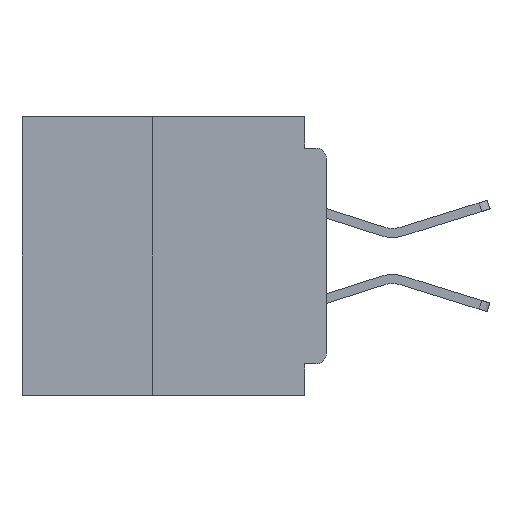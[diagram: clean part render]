
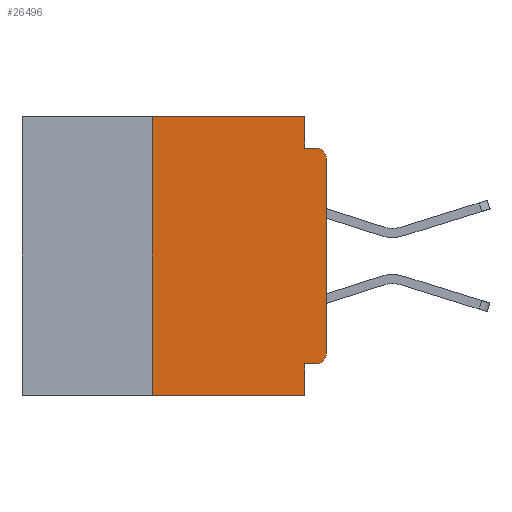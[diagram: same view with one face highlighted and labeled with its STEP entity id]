
A CAD part, left-side view. The second image highlights one B-rep face of the part: STEP entity #26496.
In plain terms, the highlighted planar face has unit normal (-1, 0, 0).
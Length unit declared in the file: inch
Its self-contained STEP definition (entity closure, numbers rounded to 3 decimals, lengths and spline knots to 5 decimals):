
#781 = LINE ( 'NONE', #15018, #24792 ) ;
#829 = CARTESIAN_POINT ( 'NONE',  ( 0., 0.015, -0.355 ) ) ;
#1220 = CARTESIAN_POINT ( 'NONE',  ( 0., 0.437, 0. ) ) ;
#1886 = EDGE_CURVE ( 'NONE', #57161, #25833, #57017, .T. ) ;
#2652 = CARTESIAN_POINT ( 'NONE',  ( 0., 0., -0.06 ) ) ;
#2807 = VERTEX_POINT ( 'NONE', #42373 ) ;
#3463 = ORIENTED_EDGE ( 'NONE', *, *, #7537, .F. ) ;
#3884 = CIRCLE ( 'NONE', #36840, 0.015 ) ;
#4123 = ORIENTED_EDGE ( 'NONE', *, *, #7112, .F. ) ;
#4292 = LINE ( 'NONE', #39189, #39430 ) ;
#5051 = CARTESIAN_POINT ( 'NONE',  ( 0., 0.031, -0.045 ) ) ;
#5560 = CARTESIAN_POINT ( 'NONE',  ( 0., 0.015, -0.34 ) ) ;
#5976 = VECTOR ( 'NONE', #29916, 39.37008 ) ;
#6452 = ORIENTED_EDGE ( 'NONE', *, *, #53035, .F. ) ;
#7112 = EDGE_CURVE ( 'NONE', #24129, #18933, #29905, .T. ) ;
#7407 = CARTESIAN_POINT ( 'NONE',  ( 0., 0., -0.34 ) ) ;
#7537 = EDGE_CURVE ( 'NONE', #20228, #24129, #18692, .T. ) ;
#7845 = PLANE ( 'NONE',  #27998 ) ;
#8189 = EDGE_CURVE ( 'NONE', #18933, #37794, #9601, .T. ) ;
#8416 = DIRECTION ( 'NONE',  ( 0., -1., 0. ) ) ;
#9601 = LINE ( 'NONE', #18985, #60178 ) ;
#9616 = LINE ( 'NONE', #17399, #20852 ) ;
#10145 = AXIS2_PLACEMENT_3D ( 'NONE', #24481, #25590, #25504 ) ;
#10401 = DIRECTION ( 'NONE',  ( 0., 0., -1. ) ) ;
#11096 = VECTOR ( 'NONE', #8416, 39.37008 ) ;
#11601 = EDGE_CURVE ( 'NONE', #55107, #50254, #9616, .T. ) ;
#13464 = CARTESIAN_POINT ( 'NONE',  ( 0., 0.437, -0.4 ) ) ;
#15018 = CARTESIAN_POINT ( 'NONE',  ( 0., 0., -0.045 ) ) ;
#15462 = DIRECTION ( 'NONE',  ( 0., 0., -1. ) ) ;
#15678 = ORIENTED_EDGE ( 'NONE', *, *, #1886, .T. ) ;
#16111 = ORIENTED_EDGE ( 'NONE', *, *, #24464, .F. ) ;
#17399 = CARTESIAN_POINT ( 'NONE',  ( 0., 0., -0.355 ) ) ;
#18692 = LINE ( 'NONE', #18847, #55066 ) ;
#18706 = ORIENTED_EDGE ( 'NONE', *, *, #11601, .F. ) ;
#18847 = CARTESIAN_POINT ( 'NONE',  ( 0., 0.25, -0.4 ) ) ;
#18933 = VERTEX_POINT ( 'NONE', #34058 ) ;
#18985 = CARTESIAN_POINT ( 'NONE',  ( 0., 0.031, 0. ) ) ;
#20228 = VERTEX_POINT ( 'NONE', #53778 ) ;
#20852 = VECTOR ( 'NONE', #41075, 39.37008 ) ;
#21966 = CARTESIAN_POINT ( 'NONE',  ( 0., 0.015, -0.045 ) ) ;
#22291 = LINE ( 'NONE', #13464, #11096 ) ;
#22297 = DIRECTION ( 'NONE',  ( 0., 0., -1. ) ) ;
#23599 = VECTOR ( 'NONE', #60745, 39.37008 ) ;
#24129 = VERTEX_POINT ( 'NONE', #32144 ) ;
#24464 = EDGE_CURVE ( 'NONE', #50254, #2807, #4292, .T. ) ;
#24481 = CARTESIAN_POINT ( 'NONE',  ( 0., 0.015, -0.06 ) ) ;
#24792 = VECTOR ( 'NONE', #53025, 39.37008 ) ;
#25103 = LINE ( 'NONE', #37173, #23599 ) ;
#25504 = DIRECTION ( 'NONE',  ( 0., 0., -1. ) ) ;
#25590 = DIRECTION ( 'NONE',  ( -1., 0., 0. ) ) ;
#25833 = VERTEX_POINT ( 'NONE', #21966 ) ;
#26496 = ADVANCED_FACE ( 'NONE', ( #38410 ), #7845, .F. ) ;
#27998 = AXIS2_PLACEMENT_3D ( 'NONE', #45972, #50729, #22297 ) ;
#28342 = EDGE_CURVE ( 'NONE', #55107, #53320, #3884, .T. ) ;
#28406 = ORIENTED_EDGE ( 'NONE', *, *, #28342, .T. ) ;
#29905 = LINE ( 'NONE', #1220, #5976 ) ;
#29916 = DIRECTION ( 'NONE',  ( 0., -1., 0. ) ) ;
#32144 = CARTESIAN_POINT ( 'NONE',  ( 0., 0.25, 0. ) ) ;
#32361 = CARTESIAN_POINT ( 'NONE',  ( 0., 0.031, -0.355 ) ) ;
#34058 = CARTESIAN_POINT ( 'NONE',  ( 0., 0.031, 0. ) ) ;
#36840 = AXIS2_PLACEMENT_3D ( 'NONE', #5560, #38963, #10401 ) ;
#37173 = CARTESIAN_POINT ( 'NONE',  ( 0., 0., 0. ) ) ;
#37794 = VERTEX_POINT ( 'NONE', #5051 ) ;
#37844 = ORIENTED_EDGE ( 'NONE', *, *, #44723, .T. ) ;
#37975 = DIRECTION ( 'NONE',  ( 0., 0., 1. ) ) ;
#38410 = FACE_OUTER_BOUND ( 'NONE', #44164, .T. ) ;
#38963 = DIRECTION ( 'NONE',  ( -1., 0., 0. ) ) ;
#39189 = CARTESIAN_POINT ( 'NONE',  ( 0., 0.031, -0.4 ) ) ;
#39430 = VECTOR ( 'NONE', #15462, 39.37008 ) ;
#41075 = DIRECTION ( 'NONE',  ( 0., 1., 0. ) ) ;
#42373 = CARTESIAN_POINT ( 'NONE',  ( 0., 0.031, -0.4 ) ) ;
#43281 = ORIENTED_EDGE ( 'NONE', *, *, #8189, .F. ) ;
#44164 = EDGE_LOOP ( 'NONE', ( #37844, #15678, #6452, #43281, #4123, #3463, #45884, #16111, #18706, #28406 ) ) ;
#44723 = EDGE_CURVE ( 'NONE', #53320, #57161, #25103, .T. ) ;
#45884 = ORIENTED_EDGE ( 'NONE', *, *, #49610, .T. ) ;
#45972 = CARTESIAN_POINT ( 'NONE',  ( 0., 0.437, 0. ) ) ;
#49610 = EDGE_CURVE ( 'NONE', #20228, #2807, #22291, .T. ) ;
#50254 = VERTEX_POINT ( 'NONE', #32361 ) ;
#50729 = DIRECTION ( 'NONE',  ( 1., 0., 0. ) ) ;
#51977 = DIRECTION ( 'NONE',  ( 0., 0., -1. ) ) ;
#53025 = DIRECTION ( 'NONE',  ( 0., -1., 0. ) ) ;
#53035 = EDGE_CURVE ( 'NONE', #37794, #25833, #781, .T. ) ;
#53320 = VERTEX_POINT ( 'NONE', #7407 ) ;
#53778 = CARTESIAN_POINT ( 'NONE',  ( 0., 0.25, -0.4 ) ) ;
#55066 = VECTOR ( 'NONE', #37975, 39.37008 ) ;
#55107 = VERTEX_POINT ( 'NONE', #829 ) ;
#57017 = CIRCLE ( 'NONE', #10145, 0.015 ) ;
#57161 = VERTEX_POINT ( 'NONE', #2652 ) ;
#60178 = VECTOR ( 'NONE', #51977, 39.37008 ) ;
#60745 = DIRECTION ( 'NONE',  ( 0., 0., 1. ) ) ;
